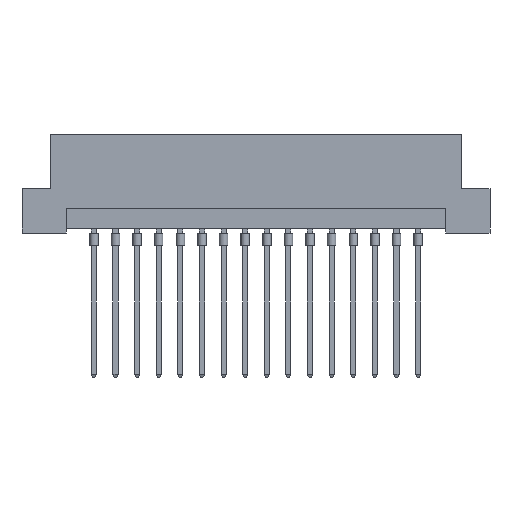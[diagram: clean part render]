
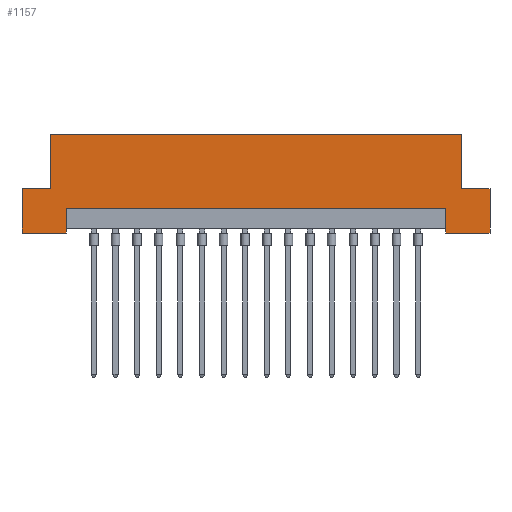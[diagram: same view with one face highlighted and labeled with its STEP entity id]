
A CAD part, front view. The second image highlights one B-rep face of the part: STEP entity #1157.
In plain terms, the highlighted planar face has unit normal (0, -1, 0).
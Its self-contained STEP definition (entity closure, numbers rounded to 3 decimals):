
#5 = DIRECTION ( 'NONE',  ( 0., 0., -1. ) ) ;
#171 = VERTEX_POINT ( 'NONE', #7601 ) ;
#193 = VERTEX_POINT ( 'NONE', #9209 ) ;
#204 = ORIENTED_EDGE ( 'NONE', *, *, #845, .F. ) ;
#226 = CARTESIAN_POINT ( 'NONE',  ( -27.5, 0., 0. ) ) ;
#236 = LINE ( 'NONE', #4300, #6342 ) ;
#338 = VERTEX_POINT ( 'NONE', #1150 ) ;
#388 = CARTESIAN_POINT ( 'NONE',  ( -22.3, 0., 0.5 ) ) ;
#484 = CARTESIAN_POINT ( 'NONE',  ( -27.5, 0., 0. ) ) ;
#796 = VECTOR ( 'NONE', #979, 1000. ) ;
#834 = CARTESIAN_POINT ( 'NONE',  ( 27.5, 0., 0. ) ) ;
#845 = EDGE_CURVE ( 'NONE', #4525, #171, #7589, .T. ) ;
#979 = DIRECTION ( 'NONE',  ( -1., 0., 0. ) ) ;
#1034 = CARTESIAN_POINT ( 'NONE',  ( 22.3, 0., 0.5 ) ) ;
#1145 = VECTOR ( 'NONE', #1387, 1000. ) ;
#1150 = CARTESIAN_POINT ( 'NONE',  ( -24.2, 0., 11.6 ) ) ;
#1157 = ADVANCED_FACE ( 'NONE', ( #1541 ), #10513, .F. ) ;
#1387 = DIRECTION ( 'NONE',  ( 0., 0., -1. ) ) ;
#1541 = FACE_OUTER_BOUND ( 'NONE', #3465, .T. ) ;
#1569 = VERTEX_POINT ( 'NONE', #8128 ) ;
#1712 = EDGE_CURVE ( 'NONE', #338, #7874, #6778, .T. ) ;
#1786 = DIRECTION ( 'NONE',  ( 1., 0., 0. ) ) ;
#1853 = EDGE_CURVE ( 'NONE', #193, #6628, #5447, .T. ) ;
#2248 = EDGE_CURVE ( 'NONE', #7413, #7874, #2643, .T. ) ;
#2291 = CARTESIAN_POINT ( 'NONE',  ( 24.2, 0., 5.2 ) ) ;
#2412 = ORIENTED_EDGE ( 'NONE', *, *, #2919, .F. ) ;
#2416 = CARTESIAN_POINT ( 'NONE',  ( -27.5, 0., 0. ) ) ;
#2556 = VERTEX_POINT ( 'NONE', #3268 ) ;
#2636 = LINE ( 'NONE', #1034, #4340 ) ;
#2640 = CARTESIAN_POINT ( 'NONE',  ( -22.3, 0., 2.9 ) ) ;
#2643 = LINE ( 'NONE', #5908, #9204 ) ;
#2919 = EDGE_CURVE ( 'NONE', #2556, #4525, #4053, .T. ) ;
#2937 = ORIENTED_EDGE ( 'NONE', *, *, #10323, .F. ) ;
#3134 = LINE ( 'NONE', #8884, #8782 ) ;
#3268 = CARTESIAN_POINT ( 'NONE',  ( 27.5, 0., 5.2 ) ) ;
#3465 = EDGE_LOOP ( 'NONE', ( #4375, #7754, #204, #2412, #5936, #5403, #9609, #2937, #5250, #7456, #10295, #4645 ) ) ;
#3618 = LINE ( 'NONE', #6734, #6879 ) ;
#3653 = DIRECTION ( 'NONE',  ( 0., 0., -1. ) ) ;
#3662 = CARTESIAN_POINT ( 'NONE',  ( -27.5, 0., 5.2 ) ) ;
#3942 = CARTESIAN_POINT ( 'NONE',  ( 24.2, 0., 11.6 ) ) ;
#3980 = VERTEX_POINT ( 'NONE', #4870 ) ;
#3991 = VERTEX_POINT ( 'NONE', #2416 ) ;
#4053 = LINE ( 'NONE', #4809, #1145 ) ;
#4300 = CARTESIAN_POINT ( 'NONE',  ( -27.5, 0., 5.2 ) ) ;
#4340 = VECTOR ( 'NONE', #5, 1000. ) ;
#4375 = ORIENTED_EDGE ( 'NONE', *, *, #1853, .F. ) ;
#4525 = VERTEX_POINT ( 'NONE', #834 ) ;
#4533 = LINE ( 'NONE', #5245, #5569 ) ;
#4645 = ORIENTED_EDGE ( 'NONE', *, *, #8352, .F. ) ;
#4704 = DIRECTION ( 'NONE',  ( 0., 1., 0. ) ) ;
#4787 = DIRECTION ( 'NONE',  ( 1., 0., 0. ) ) ;
#4808 = VERTEX_POINT ( 'NONE', #3662 ) ;
#4809 = CARTESIAN_POINT ( 'NONE',  ( 27.5, 0., 0. ) ) ;
#4870 = CARTESIAN_POINT ( 'NONE',  ( -24.2, 0., 5.2 ) ) ;
#5245 = CARTESIAN_POINT ( 'NONE',  ( -27.5, 0., 0. ) ) ;
#5250 = ORIENTED_EDGE ( 'NONE', *, *, #6249, .F. ) ;
#5264 = AXIS2_PLACEMENT_3D ( 'NONE', #7303, #4704, #5485 ) ;
#5403 = ORIENTED_EDGE ( 'NONE', *, *, #2248, .T. ) ;
#5447 = LINE ( 'NONE', #6949, #5781 ) ;
#5485 = DIRECTION ( 'NONE',  ( 0., 0., 1. ) ) ;
#5569 = VECTOR ( 'NONE', #10191, 1000. ) ;
#5781 = VECTOR ( 'NONE', #7119, 1000. ) ;
#5873 = CARTESIAN_POINT ( 'NONE',  ( -27.5, 0., 11.6 ) ) ;
#5908 = CARTESIAN_POINT ( 'NONE',  ( 24.2, 0., 5.2 ) ) ;
#5936 = ORIENTED_EDGE ( 'NONE', *, *, #9144, .F. ) ;
#6049 = LINE ( 'NONE', #484, #6830 ) ;
#6066 = LINE ( 'NONE', #388, #6444 ) ;
#6249 = EDGE_CURVE ( 'NONE', #4808, #3980, #236, .T. ) ;
#6342 = VECTOR ( 'NONE', #7599, 1000. ) ;
#6444 = VECTOR ( 'NONE', #3653, 1000. ) ;
#6628 = VERTEX_POINT ( 'NONE', #2640 ) ;
#6734 = CARTESIAN_POINT ( 'NONE',  ( -24.2, 0., 5.2 ) ) ;
#6778 = LINE ( 'NONE', #5873, #8870 ) ;
#6830 = VECTOR ( 'NONE', #7039, 1000. ) ;
#6879 = VECTOR ( 'NONE', #10012, 1000. ) ;
#6949 = CARTESIAN_POINT ( 'NONE',  ( 22.3, 0., 2.9 ) ) ;
#7039 = DIRECTION ( 'NONE',  ( 0., 0., 1. ) ) ;
#7119 = DIRECTION ( 'NONE',  ( -1., 0., 0. ) ) ;
#7171 = EDGE_CURVE ( 'NONE', #3991, #4808, #6049, .T. ) ;
#7303 = CARTESIAN_POINT ( 'NONE',  ( -27.5, 0., 11.6 ) ) ;
#7413 = VERTEX_POINT ( 'NONE', #2291 ) ;
#7456 = ORIENTED_EDGE ( 'NONE', *, *, #7171, .F. ) ;
#7589 = LINE ( 'NONE', #226, #796 ) ;
#7599 = DIRECTION ( 'NONE',  ( 1., 0., 0. ) ) ;
#7601 = CARTESIAN_POINT ( 'NONE',  ( 22.3, 0., 0. ) ) ;
#7754 = ORIENTED_EDGE ( 'NONE', *, *, #9764, .T. ) ;
#7874 = VERTEX_POINT ( 'NONE', #3942 ) ;
#8128 = CARTESIAN_POINT ( 'NONE',  ( -22.3, 0., 0. ) ) ;
#8352 = EDGE_CURVE ( 'NONE', #6628, #1569, #6066, .T. ) ;
#8782 = VECTOR ( 'NONE', #4787, 1000. ) ;
#8835 = EDGE_CURVE ( 'NONE', #1569, #3991, #4533, .T. ) ;
#8870 = VECTOR ( 'NONE', #1786, 1000. ) ;
#8884 = CARTESIAN_POINT ( 'NONE',  ( 27.5, 0., 5.2 ) ) ;
#9144 = EDGE_CURVE ( 'NONE', #7413, #2556, #3134, .T. ) ;
#9204 = VECTOR ( 'NONE', #10362, 1000. ) ;
#9209 = CARTESIAN_POINT ( 'NONE',  ( 22.3, 0., 2.9 ) ) ;
#9609 = ORIENTED_EDGE ( 'NONE', *, *, #1712, .F. ) ;
#9764 = EDGE_CURVE ( 'NONE', #193, #171, #2636, .T. ) ;
#10012 = DIRECTION ( 'NONE',  ( 0., 0., 1. ) ) ;
#10191 = DIRECTION ( 'NONE',  ( -1., 0., 0. ) ) ;
#10295 = ORIENTED_EDGE ( 'NONE', *, *, #8835, .F. ) ;
#10323 = EDGE_CURVE ( 'NONE', #3980, #338, #3618, .T. ) ;
#10362 = DIRECTION ( 'NONE',  ( 0., 0., 1. ) ) ;
#10513 = PLANE ( 'NONE',  #5264 ) ;
